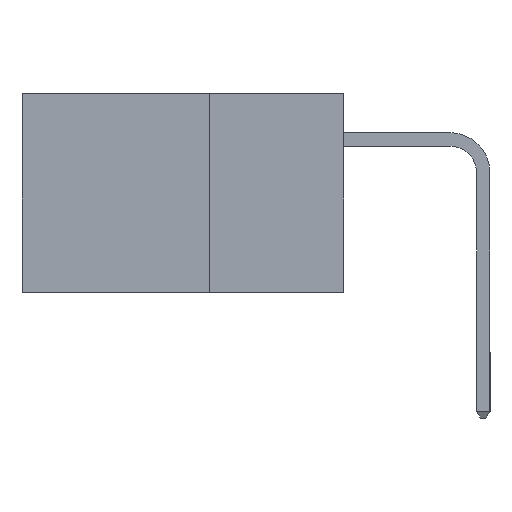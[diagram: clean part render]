
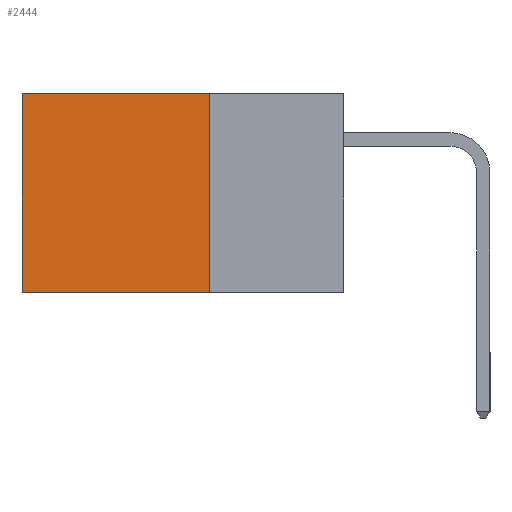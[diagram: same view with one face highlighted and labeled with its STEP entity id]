
A CAD part, left-side view. The second image highlights one B-rep face of the part: STEP entity #2444.
In plain terms, the highlighted planar face has unit normal (-1, 0, 0).
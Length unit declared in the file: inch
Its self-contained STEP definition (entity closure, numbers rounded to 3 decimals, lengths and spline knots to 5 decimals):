
#414 = CARTESIAN_POINT ( 'NONE',  ( 0.298, 0.25, -0.37 ) ) ;
#1370 = EDGE_CURVE ( 'NONE', #24549, #17535, #3106, .T. ) ;
#2120 = DIRECTION ( 'NONE',  ( 0., 0., -1. ) ) ;
#2147 = VECTOR ( 'NONE', #2120, 39.37008 ) ;
#2444 = ADVANCED_FACE ( 'NONE', ( #26537 ), #11507, .F. ) ;
#2644 = ORIENTED_EDGE ( 'NONE', *, *, #15315, .F. ) ;
#3067 = DIRECTION ( 'NONE',  ( 1., 0., 0. ) ) ;
#3106 = LINE ( 'NONE', #24788, #2147 ) ;
#3146 = CARTESIAN_POINT ( 'NONE',  ( 0.298, 0.25, 0. ) ) ;
#5199 = ORIENTED_EDGE ( 'NONE', *, *, #1370, .F. ) ;
#7523 = DIRECTION ( 'NONE',  ( 0., 1., 0. ) ) ;
#8149 = ORIENTED_EDGE ( 'NONE', *, *, #13967, .T. ) ;
#9302 = VERTEX_POINT ( 'NONE', #13388 ) ;
#9613 = LINE ( 'NONE', #9694, #14513 ) ;
#9694 = CARTESIAN_POINT ( 'NONE',  ( 0.298, 0.6, 0. ) ) ;
#10092 = EDGE_CURVE ( 'NONE', #22004, #9302, #9613, .T. ) ;
#11419 = DIRECTION ( 'NONE',  ( 0., 0., -1. ) ) ;
#11507 = PLANE ( 'NONE',  #11511 ) ;
#11511 = AXIS2_PLACEMENT_3D ( 'NONE', #11703, #3067, #11419 ) ;
#11703 = CARTESIAN_POINT ( 'NONE',  ( 0.298, 0.25, 0. ) ) ;
#11766 = VECTOR ( 'NONE', #7523, 39.37008 ) ;
#11923 = EDGE_LOOP ( 'NONE', ( #26394, #2644, #5199, #8149 ) ) ;
#13388 = CARTESIAN_POINT ( 'NONE',  ( 0.298, 0.6, -0.37 ) ) ;
#13967 = EDGE_CURVE ( 'NONE', #24549, #22004, #15054, .T. ) ;
#14454 = CARTESIAN_POINT ( 'NONE',  ( 0.298, 0.6, 0. ) ) ;
#14513 = VECTOR ( 'NONE', #20618, 39.37008 ) ;
#15054 = LINE ( 'NONE', #3146, #11766 ) ;
#15315 = EDGE_CURVE ( 'NONE', #17535, #9302, #21182, .T. ) ;
#15881 = CARTESIAN_POINT ( 'NONE',  ( 0.298, 0.25, -0.37 ) ) ;
#17535 = VERTEX_POINT ( 'NONE', #414 ) ;
#20618 = DIRECTION ( 'NONE',  ( 0., 0., -1. ) ) ;
#21182 = LINE ( 'NONE', #15881, #26075 ) ;
#22004 = VERTEX_POINT ( 'NONE', #14454 ) ;
#24549 = VERTEX_POINT ( 'NONE', #26844 ) ;
#24788 = CARTESIAN_POINT ( 'NONE',  ( 0.298, 0.25, 0. ) ) ;
#26075 = VECTOR ( 'NONE', #26161, 39.37008 ) ;
#26161 = DIRECTION ( 'NONE',  ( 0., 1., 0. ) ) ;
#26394 = ORIENTED_EDGE ( 'NONE', *, *, #10092, .T. ) ;
#26537 = FACE_OUTER_BOUND ( 'NONE', #11923, .T. ) ;
#26844 = CARTESIAN_POINT ( 'NONE',  ( 0.298, 0.25, 0. ) ) ;
